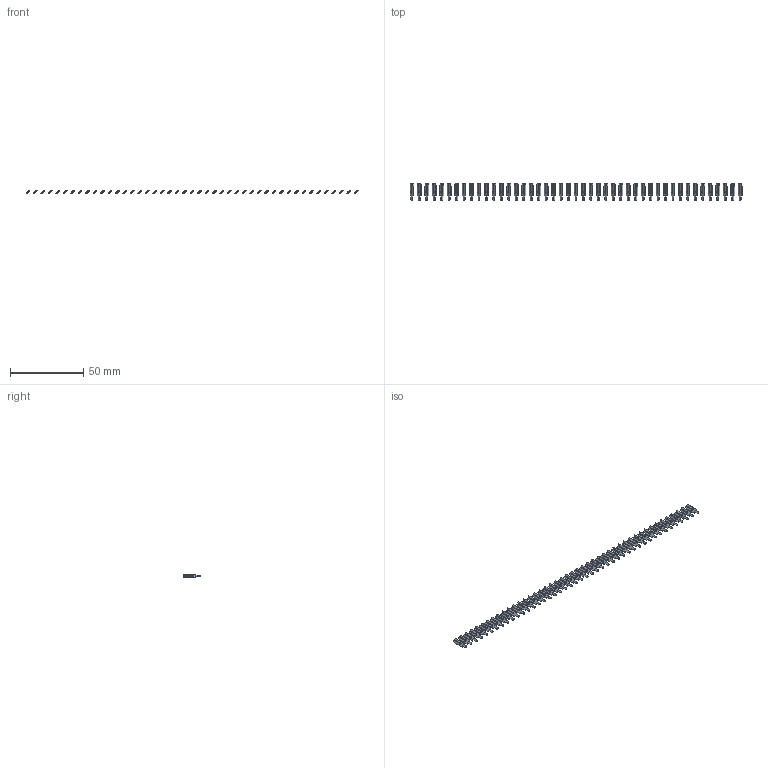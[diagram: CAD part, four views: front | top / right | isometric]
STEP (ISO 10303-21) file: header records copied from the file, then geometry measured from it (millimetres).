
FILE_DESCRIPTION (( 'STEP AP203' ), '1' );
FILE_NAME ('106-045-250-200.STEP', '2020-04-16T20:22:33', ( '' ), ( '' ), 'SwSTEP 2.0', 'SolidWorks 2016', '' );
FILE_SCHEMA (( 'CONFIG_CONTROL_DESIGN' ));
Length unit declared in the file: inch
Products named in the file (2): 106-045-250-200; 100-290-001_100-290-250
Assembly tree (45 placements, depth 2):
  106-045-250-200
    100-290-001_100-290-250  x45
Bounding box: 226.05 x 11.48 x 2.53 mm (x, y, z)
Volume: 702.2 mm3; surface area: 3300.7 mm2
Topology: 45 solids, 45 shells, 1080 faces, 2970 edges, 1980 vertices
Faces by surface type: plane 900, cylinder 180
Entity records: 2366 total; most frequent: DIRECTION 214, CARTESIAN_POINT 194, ORIENTED_EDGE 132, COORDINATED_UNIVERSAL_TIME_OFFSET 100, LOCAL_TIME 100, DATE_AND_TIME 100, CALENDAR_DATE 100, AXIS2_PLACEMENT_3D 80
